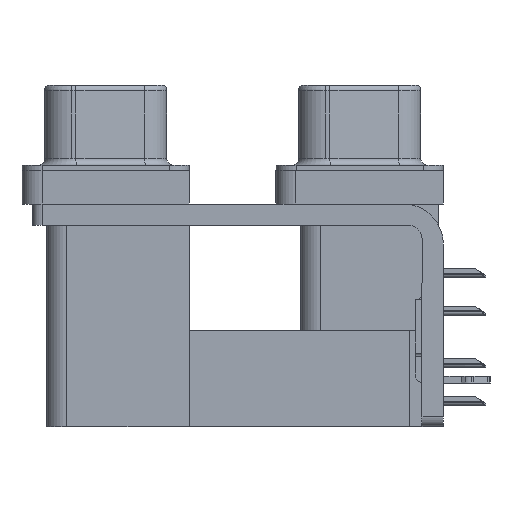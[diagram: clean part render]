
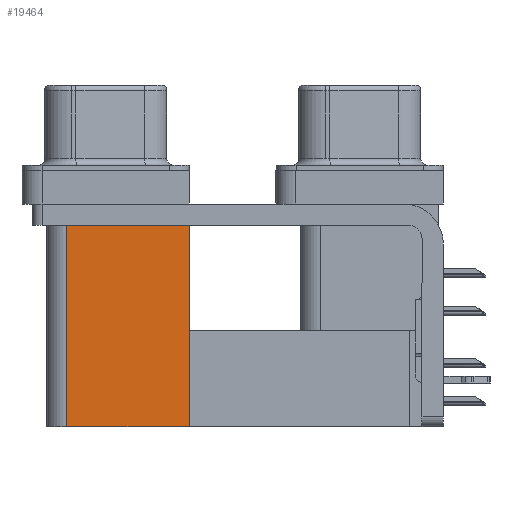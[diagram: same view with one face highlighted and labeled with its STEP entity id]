
A CAD part, left-side view. The second image highlights one B-rep face of the part: STEP entity #19464.
In plain terms, the highlighted planar face has unit normal (-1, 0, 0).
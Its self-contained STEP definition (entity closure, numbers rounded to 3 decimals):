
#597 = ORIENTED_EDGE ( 'NONE', *, *, #26203, .T. ) ;
#1369 = VECTOR ( 'NONE', #2354, 1000. ) ;
#2348 = AXIS2_PLACEMENT_3D ( 'NONE', #39023, #4177, #19677 ) ;
#2354 = DIRECTION ( 'NONE',  ( 0., 0., 1. ) ) ;
#4177 = DIRECTION ( 'NONE',  ( 1., 0., 0. ) ) ;
#7765 = DIRECTION ( 'NONE',  ( 0., 0., 1. ) ) ;
#8001 = PLANE ( 'NONE',  #2348 ) ;
#11643 = VERTEX_POINT ( 'NONE', #26798 ) ;
#12378 = VERTEX_POINT ( 'NONE', #16181 ) ;
#12680 = CARTESIAN_POINT ( 'NONE',  ( 3.79, 12.775, -19.2 ) ) ;
#13638 = CARTESIAN_POINT ( 'NONE',  ( 3.79, 12.775, -19.2 ) ) ;
#16181 = CARTESIAN_POINT ( 'NONE',  ( 3.79, 12.775, -2.5 ) ) ;
#16587 = ORIENTED_EDGE ( 'NONE', *, *, #30535, .F. ) ;
#17833 = CARTESIAN_POINT ( 'NONE',  ( 3.79, 12.775, -2.5 ) ) ;
#19464 = ADVANCED_FACE ( 'NONE', ( #42837 ), #8001, .F. ) ;
#19677 = DIRECTION ( 'NONE',  ( 0., 0., -1. ) ) ;
#23401 = LINE ( 'NONE', #12680, #33560 ) ;
#23555 = EDGE_CURVE ( 'NONE', #31160, #12378, #34981, .T. ) ;
#25711 = LINE ( 'NONE', #17833, #31984 ) ;
#25741 = LINE ( 'NONE', #29317, #1369 ) ;
#25818 = EDGE_LOOP ( 'NONE', ( #597, #34204, #16587, #34175 ) ) ;
#25981 = DIRECTION ( 'NONE',  ( 0., 1., 0. ) ) ;
#26203 = EDGE_CURVE ( 'NONE', #12378, #11643, #25711, .T. ) ;
#26798 = CARTESIAN_POINT ( 'NONE',  ( 3.79, 21.975, -2.5 ) ) ;
#29317 = CARTESIAN_POINT ( 'NONE',  ( 3.79, 21.975, -19.2 ) ) ;
#29348 = VECTOR ( 'NONE', #7765, 1000. ) ;
#30535 = EDGE_CURVE ( 'NONE', #31160, #36122, #23401, .T. ) ;
#31160 = VERTEX_POINT ( 'NONE', #13638 ) ;
#31984 = VECTOR ( 'NONE', #25981, 1000. ) ;
#33560 = VECTOR ( 'NONE', #35848, 1000. ) ;
#34175 = ORIENTED_EDGE ( 'NONE', *, *, #23555, .T. ) ;
#34204 = ORIENTED_EDGE ( 'NONE', *, *, #46598, .F. ) ;
#34981 = LINE ( 'NONE', #47182, #29348 ) ;
#35848 = DIRECTION ( 'NONE',  ( 0., 1., 0. ) ) ;
#36122 = VERTEX_POINT ( 'NONE', #49429 ) ;
#39023 = CARTESIAN_POINT ( 'NONE',  ( 3.79, 12.775, -19.2 ) ) ;
#42837 = FACE_OUTER_BOUND ( 'NONE', #25818, .T. ) ;
#46598 = EDGE_CURVE ( 'NONE', #36122, #11643, #25741, .T. ) ;
#47182 = CARTESIAN_POINT ( 'NONE',  ( 3.79, 12.775, -19.2 ) ) ;
#49429 = CARTESIAN_POINT ( 'NONE',  ( 3.79, 21.975, -19.2 ) ) ;
